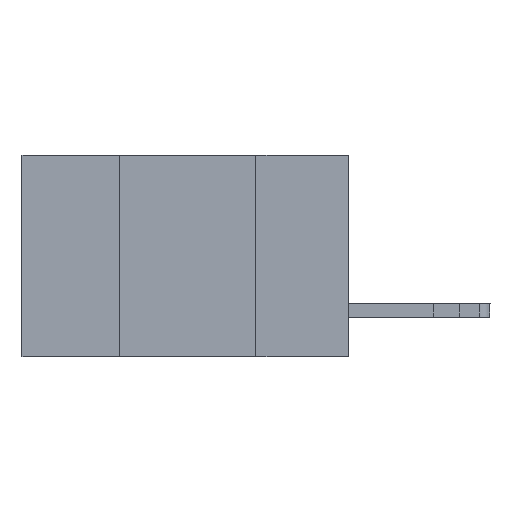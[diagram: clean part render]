
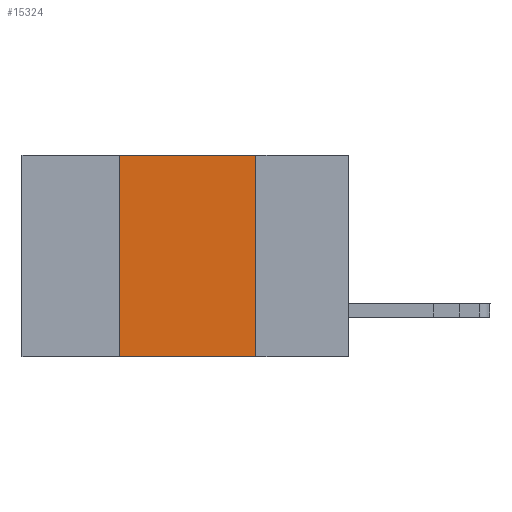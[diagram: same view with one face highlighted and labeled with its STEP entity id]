
A CAD part, left-side view. The second image highlights one B-rep face of the part: STEP entity #15324.
In plain terms, the highlighted planar face has unit normal (-1, 0, 0).
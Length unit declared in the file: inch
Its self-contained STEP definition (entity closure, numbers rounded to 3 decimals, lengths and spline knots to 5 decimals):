
#1732 = EDGE_CURVE ( 'NONE', #8220, #15655, #16661, .T. ) ;
#2655 = VERTEX_POINT ( 'NONE', #12060 ) ;
#2861 = EDGE_CURVE ( 'NONE', #11259, #2655, #13084, .T. ) ;
#4104 = DIRECTION ( 'NONE',  ( 0., -1., 0. ) ) ;
#4175 = CARTESIAN_POINT ( 'NONE',  ( 0., 0.6, -0.37 ) ) ;
#5472 = EDGE_CURVE ( 'NONE', #8220, #11259, #14647, .T. ) ;
#7014 = DIRECTION ( 'NONE',  ( 1., 0., 0. ) ) ;
#7871 = CARTESIAN_POINT ( 'NONE',  ( 0., 0.42, -0.37 ) ) ;
#7877 = VECTOR ( 'NONE', #15958, 39.37008 ) ;
#8220 = VERTEX_POINT ( 'NONE', #11124 ) ;
#9725 = PLANE ( 'NONE',  #11077 ) ;
#9921 = DIRECTION ( 'NONE',  ( 0., -1., 0. ) ) ;
#9936 = VECTOR ( 'NONE', #4104, 39.37008 ) ;
#9937 = CARTESIAN_POINT ( 'NONE',  ( 0., 0.6, 0. ) ) ;
#9945 = ORIENTED_EDGE ( 'NONE', *, *, #5472, .F. ) ;
#10224 = EDGE_LOOP ( 'NONE', ( #14790, #13484, #9945, #14371 ) ) ;
#10478 = CARTESIAN_POINT ( 'NONE',  ( 0., 0.17, -0.37 ) ) ;
#10502 = EDGE_CURVE ( 'NONE', #2655, #15655, #17295, .T. ) ;
#11077 = AXIS2_PLACEMENT_3D ( 'NONE', #12445, #7014, #16472 ) ;
#11124 = CARTESIAN_POINT ( 'NONE',  ( 0., 0.42, -0.37 ) ) ;
#11259 = VERTEX_POINT ( 'NONE', #16598 ) ;
#12060 = CARTESIAN_POINT ( 'NONE',  ( 0., 0.17, 0. ) ) ;
#12350 = CARTESIAN_POINT ( 'NONE',  ( 0., 0.17, -0.37 ) ) ;
#12445 = CARTESIAN_POINT ( 'NONE',  ( 0., 0.6, 0. ) ) ;
#13084 = LINE ( 'NONE', #9937, #16623 ) ;
#13484 = ORIENTED_EDGE ( 'NONE', *, *, #2861, .F. ) ;
#13772 = VECTOR ( 'NONE', #17722, 39.37008 ) ;
#14371 = ORIENTED_EDGE ( 'NONE', *, *, #1732, .T. ) ;
#14647 = LINE ( 'NONE', #7871, #7877 ) ;
#14790 = ORIENTED_EDGE ( 'NONE', *, *, #10502, .F. ) ;
#15324 = ADVANCED_FACE ( 'NONE', ( #15609 ), #9725, .F. ) ;
#15609 = FACE_OUTER_BOUND ( 'NONE', #10224, .T. ) ;
#15655 = VERTEX_POINT ( 'NONE', #10478 ) ;
#15958 = DIRECTION ( 'NONE',  ( 0., 0., 1. ) ) ;
#16472 = DIRECTION ( 'NONE',  ( 0., 0., -1. ) ) ;
#16598 = CARTESIAN_POINT ( 'NONE',  ( 0., 0.42, 0. ) ) ;
#16623 = VECTOR ( 'NONE', #9921, 39.37008 ) ;
#16661 = LINE ( 'NONE', #4175, #9936 ) ;
#17295 = LINE ( 'NONE', #12350, #13772 ) ;
#17722 = DIRECTION ( 'NONE',  ( 0., 0., -1. ) ) ;
